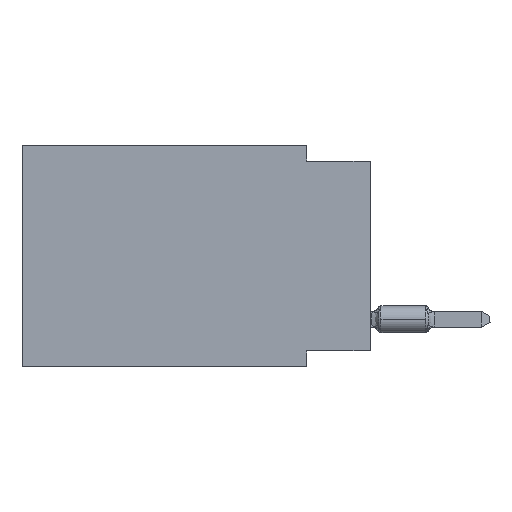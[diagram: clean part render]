
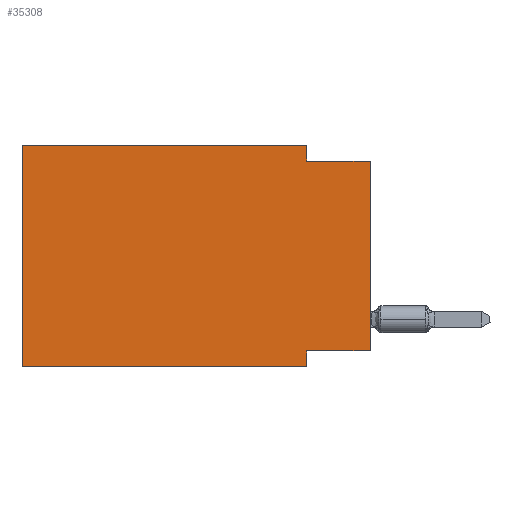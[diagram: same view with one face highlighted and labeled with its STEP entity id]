
A CAD part, left-side view. The second image highlights one B-rep face of the part: STEP entity #35308.
In plain terms, the highlighted planar face has unit normal (-1, 0, 0).
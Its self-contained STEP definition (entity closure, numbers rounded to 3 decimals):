
#1458 = EDGE_LOOP ( 'NONE', ( #28165, #12707, #34918, #42792, #21665, #29937, #21707, #26696 ) ) ;
#1921 = EDGE_CURVE ( 'NONE', #27398, #2352, #12943, .T. ) ;
#2352 = VERTEX_POINT ( 'NONE', #8787 ) ;
#2932 = DIRECTION ( 'NONE',  ( 0., 0., -1. ) ) ;
#3379 = LINE ( 'NONE', #16772, #33998 ) ;
#4719 = VERTEX_POINT ( 'NONE', #41008 ) ;
#5430 = LINE ( 'NONE', #12137, #13843 ) ;
#5913 = DIRECTION ( 'NONE',  ( 0., 0., 1. ) ) ;
#5997 = CARTESIAN_POINT ( 'NONE',  ( 0., 13.97, 0. ) ) ;
#7386 = VECTOR ( 'NONE', #37792, 1000. ) ;
#8412 = VECTOR ( 'NONE', #25467, 1000. ) ;
#8622 = CARTESIAN_POINT ( 'NONE',  ( 0., 0., -8.255 ) ) ;
#8787 = CARTESIAN_POINT ( 'NONE',  ( 0., 2.54, -8.255 ) ) ;
#10138 = VERTEX_POINT ( 'NONE', #13462 ) ;
#10679 = CARTESIAN_POINT ( 'NONE',  ( 0., 2.54, 0. ) ) ;
#11351 = AXIS2_PLACEMENT_3D ( 'NONE', #30639, #37352, #17429 ) ;
#12137 = CARTESIAN_POINT ( 'NONE',  ( 0., 0., -0.635 ) ) ;
#12707 = ORIENTED_EDGE ( 'NONE', *, *, #14374, .F. ) ;
#12943 = LINE ( 'NONE', #8622, #16415 ) ;
#13462 = CARTESIAN_POINT ( 'NONE',  ( 0., 2.54, -8.89 ) ) ;
#13695 = DIRECTION ( 'NONE',  ( 0., 0., -1. ) ) ;
#13843 = VECTOR ( 'NONE', #22300, 1000. ) ;
#13965 = PLANE ( 'NONE',  #11351 ) ;
#14374 = EDGE_CURVE ( 'NONE', #22889, #27222, #5430, .T. ) ;
#14622 = CARTESIAN_POINT ( 'NONE',  ( 0., 0., 0. ) ) ;
#16401 = EDGE_CURVE ( 'NONE', #2352, #10138, #18733, .T. ) ;
#16415 = VECTOR ( 'NONE', #21820, 1000. ) ;
#16772 = CARTESIAN_POINT ( 'NONE',  ( 0., 13.97, -8.89 ) ) ;
#17429 = DIRECTION ( 'NONE',  ( 0., 0., -1. ) ) ;
#17840 = EDGE_CURVE ( 'NONE', #27398, #27222, #28474, .T. ) ;
#17892 = CARTESIAN_POINT ( 'NONE',  ( 0., 2.54, 0. ) ) ;
#18127 = VECTOR ( 'NONE', #13695, 1000. ) ;
#18733 = LINE ( 'NONE', #19377, #23253 ) ;
#19377 = CARTESIAN_POINT ( 'NONE',  ( 0., 2.54, -8.89 ) ) ;
#20567 = VERTEX_POINT ( 'NONE', #22752 ) ;
#21564 = CARTESIAN_POINT ( 'NONE',  ( 0., 0., -8.255 ) ) ;
#21665 = ORIENTED_EDGE ( 'NONE', *, *, #32868, .F. ) ;
#21707 = ORIENTED_EDGE ( 'NONE', *, *, #16401, .F. ) ;
#21820 = DIRECTION ( 'NONE',  ( 0., 1., 0. ) ) ;
#22300 = DIRECTION ( 'NONE',  ( 0., -1., 0. ) ) ;
#22631 = VERTEX_POINT ( 'NONE', #17892 ) ;
#22752 = CARTESIAN_POINT ( 'NONE',  ( 0., 13.97, -8.89 ) ) ;
#22889 = VERTEX_POINT ( 'NONE', #31746 ) ;
#23253 = VECTOR ( 'NONE', #2932, 1000. ) ;
#25467 = DIRECTION ( 'NONE',  ( 0., -1., 0. ) ) ;
#25804 = LINE ( 'NONE', #35561, #27876 ) ;
#26209 = CARTESIAN_POINT ( 'NONE',  ( 0., 0., -0.635 ) ) ;
#26311 = EDGE_CURVE ( 'NONE', #22631, #22889, #30165, .T. ) ;
#26696 = ORIENTED_EDGE ( 'NONE', *, *, #1921, .F. ) ;
#27222 = VERTEX_POINT ( 'NONE', #26209 ) ;
#27398 = VERTEX_POINT ( 'NONE', #21564 ) ;
#27876 = VECTOR ( 'NONE', #5913, 1000. ) ;
#28165 = ORIENTED_EDGE ( 'NONE', *, *, #17840, .T. ) ;
#28474 = LINE ( 'NONE', #14622, #7386 ) ;
#29492 = EDGE_CURVE ( 'NONE', #4719, #22631, #31955, .T. ) ;
#29611 = EDGE_CURVE ( 'NONE', #20567, #10138, #3379, .T. ) ;
#29937 = ORIENTED_EDGE ( 'NONE', *, *, #29611, .T. ) ;
#30165 = LINE ( 'NONE', #10679, #18127 ) ;
#30639 = CARTESIAN_POINT ( 'NONE',  ( 0., 13.97, 0. ) ) ;
#30848 = FACE_OUTER_BOUND ( 'NONE', #1458, .T. ) ;
#31746 = CARTESIAN_POINT ( 'NONE',  ( 0., 2.54, -0.635 ) ) ;
#31955 = LINE ( 'NONE', #5997, #8412 ) ;
#32868 = EDGE_CURVE ( 'NONE', #20567, #4719, #25804, .T. ) ;
#33998 = VECTOR ( 'NONE', #40152, 1000. ) ;
#34918 = ORIENTED_EDGE ( 'NONE', *, *, #26311, .F. ) ;
#35308 = ADVANCED_FACE ( 'NONE', ( #30848 ), #13965, .F. ) ;
#35561 = CARTESIAN_POINT ( 'NONE',  ( 0., 13.97, 0. ) ) ;
#37352 = DIRECTION ( 'NONE',  ( 1., 0., 0. ) ) ;
#37792 = DIRECTION ( 'NONE',  ( 0., 0., 1. ) ) ;
#40152 = DIRECTION ( 'NONE',  ( 0., -1., 0. ) ) ;
#41008 = CARTESIAN_POINT ( 'NONE',  ( 0., 13.97, 0. ) ) ;
#42792 = ORIENTED_EDGE ( 'NONE', *, *, #29492, .F. ) ;
